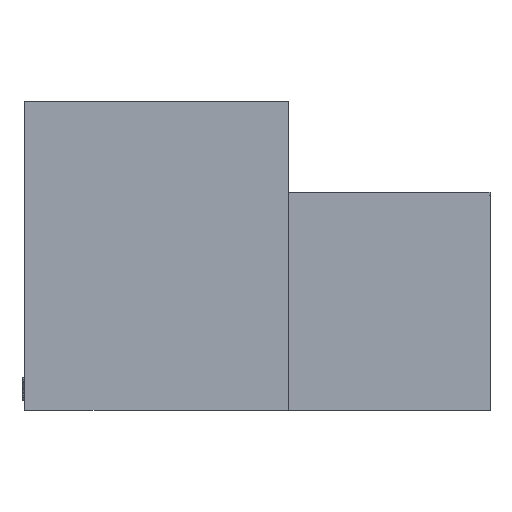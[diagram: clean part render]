
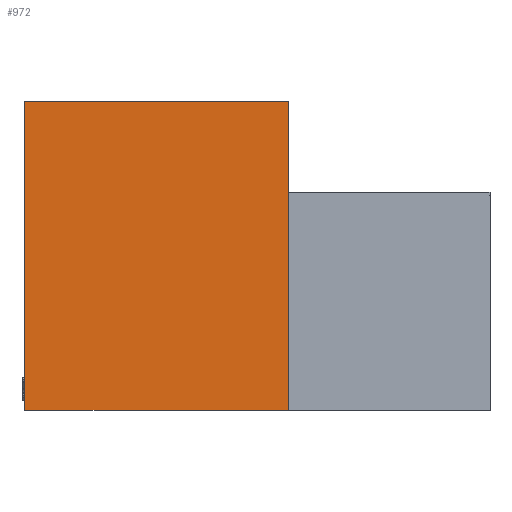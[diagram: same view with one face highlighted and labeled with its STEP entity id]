
A CAD part, left-side view. The second image highlights one B-rep face of the part: STEP entity #972.
In plain terms, the highlighted planar face has unit normal (-1, 0, 0).
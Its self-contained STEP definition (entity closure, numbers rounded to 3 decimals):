
#107 = DIRECTION ( 'NONE',  ( 0., 0., 1. ) ) ;
#294 = PLANE ( 'NONE',  #11643 ) ;
#892 = ORIENTED_EDGE ( 'NONE', *, *, #7996, .F. ) ;
#972 = ADVANCED_FACE ( 'NONE', ( #18535 ), #294, .F. ) ;
#3995 = EDGE_CURVE ( 'NONE', #17701, #9900, #5898, .T. ) ;
#4169 = ORIENTED_EDGE ( 'NONE', *, *, #17115, .F. ) ;
#4354 = VECTOR ( 'NONE', #6893, 1000. ) ;
#5393 = LINE ( 'NONE', #19348, #7892 ) ;
#5898 = LINE ( 'NONE', #7059, #4354 ) ;
#6708 = CARTESIAN_POINT ( 'NONE',  ( 0., 11.506, 0. ) ) ;
#6893 = DIRECTION ( 'NONE',  ( 0., -1., 0. ) ) ;
#7059 = CARTESIAN_POINT ( 'NONE',  ( 0., 11.506, 0. ) ) ;
#7066 = CARTESIAN_POINT ( 'NONE',  ( 0., 0., 0. ) ) ;
#7350 = EDGE_CURVE ( 'NONE', #9900, #17515, #5393, .T. ) ;
#7892 = VECTOR ( 'NONE', #11279, 1000. ) ;
#7996 = EDGE_CURVE ( 'NONE', #17515, #20058, #16339, .T. ) ;
#8421 = ORIENTED_EDGE ( 'NONE', *, *, #7350, .F. ) ;
#9900 = VERTEX_POINT ( 'NONE', #7066 ) ;
#11022 = VECTOR ( 'NONE', #24589, 1000. ) ;
#11085 = ORIENTED_EDGE ( 'NONE', *, *, #3995, .F. ) ;
#11279 = DIRECTION ( 'NONE',  ( 0., 0., -1. ) ) ;
#11643 = AXIS2_PLACEMENT_3D ( 'NONE', #20342, #18481, #24502 ) ;
#12090 = CARTESIAN_POINT ( 'NONE',  ( 0., 11.506, -13.487 ) ) ;
#16339 = LINE ( 'NONE', #24416, #11022 ) ;
#17115 = EDGE_CURVE ( 'NONE', #20058, #17701, #25538, .T. ) ;
#17515 = VERTEX_POINT ( 'NONE', #18369 ) ;
#17701 = VERTEX_POINT ( 'NONE', #6708 ) ;
#18369 = CARTESIAN_POINT ( 'NONE',  ( 0., 0., -13.487 ) ) ;
#18481 = DIRECTION ( 'NONE',  ( 1., 0., 0. ) ) ;
#18535 = FACE_OUTER_BOUND ( 'NONE', #22893, .T. ) ;
#19348 = CARTESIAN_POINT ( 'NONE',  ( 0., 0., 0. ) ) ;
#20058 = VERTEX_POINT ( 'NONE', #24905 ) ;
#20222 = VECTOR ( 'NONE', #107, 1000. ) ;
#20342 = CARTESIAN_POINT ( 'NONE',  ( 0., 0., 0. ) ) ;
#22893 = EDGE_LOOP ( 'NONE', ( #892, #8421, #11085, #4169 ) ) ;
#24416 = CARTESIAN_POINT ( 'NONE',  ( 0., -8.814, -13.487 ) ) ;
#24502 = DIRECTION ( 'NONE',  ( 0., 0., -1. ) ) ;
#24589 = DIRECTION ( 'NONE',  ( 0., 1., 0. ) ) ;
#24905 = CARTESIAN_POINT ( 'NONE',  ( 0., 11.506, -13.487 ) ) ;
#25538 = LINE ( 'NONE', #12090, #20222 ) ;
